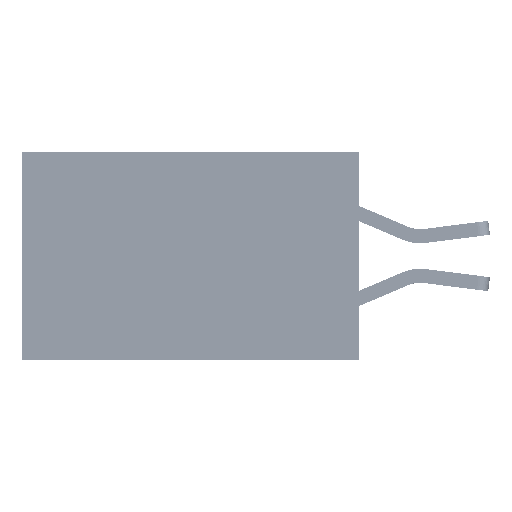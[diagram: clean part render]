
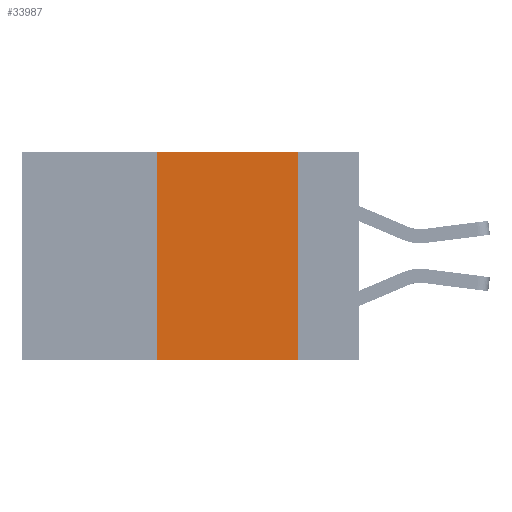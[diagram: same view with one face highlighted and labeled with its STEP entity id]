
A CAD part, left-side view. The second image highlights one B-rep face of the part: STEP entity #33987.
In plain terms, the highlighted planar face has unit normal (-1, 0, 0).
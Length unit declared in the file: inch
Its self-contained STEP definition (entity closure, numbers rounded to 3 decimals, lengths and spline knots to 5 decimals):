
#4740 = LINE ( 'NONE', #5862, #39469 ) ;
#4806 = LINE ( 'NONE', #19935, #34744 ) ;
#5862 = CARTESIAN_POINT ( 'NONE',  ( 0., 0.6, -0.37 ) ) ;
#6550 = CARTESIAN_POINT ( 'NONE',  ( 0., 0.11, -0.37 ) ) ;
#7282 = VECTOR ( 'NONE', #29513, 39.37008 ) ;
#7959 = VERTEX_POINT ( 'NONE', #6550 ) ;
#8239 = CARTESIAN_POINT ( 'NONE',  ( 0., 0.36, 0. ) ) ;
#9688 = VECTOR ( 'NONE', #29973, 39.37008 ) ;
#13762 = VERTEX_POINT ( 'NONE', #41750 ) ;
#14531 = CARTESIAN_POINT ( 'NONE',  ( 0., 0.11, 0. ) ) ;
#14538 = ORIENTED_EDGE ( 'NONE', *, *, #48262, .F. ) ;
#15694 = AXIS2_PLACEMENT_3D ( 'NONE', #31731, #24053, #27893 ) ;
#19935 = CARTESIAN_POINT ( 'NONE',  ( 0., 0.6, 0. ) ) ;
#20183 = PLANE ( 'NONE',  #15694 ) ;
#22942 = ORIENTED_EDGE ( 'NONE', *, *, #47443, .F. ) ;
#24053 = DIRECTION ( 'NONE',  ( 1., 0., 0. ) ) ;
#26331 = ORIENTED_EDGE ( 'NONE', *, *, #41389, .T. ) ;
#26552 = FACE_OUTER_BOUND ( 'NONE', #44270, .T. ) ;
#27893 = DIRECTION ( 'NONE',  ( 0., 0., -1. ) ) ;
#29513 = DIRECTION ( 'NONE',  ( 0., 0., 1. ) ) ;
#29973 = DIRECTION ( 'NONE',  ( 0., 0., -1. ) ) ;
#31731 = CARTESIAN_POINT ( 'NONE',  ( 0., 0.6, 0. ) ) ;
#32965 = VERTEX_POINT ( 'NONE', #38809 ) ;
#33987 = ADVANCED_FACE ( 'NONE', ( #26552 ), #20183, .F. ) ;
#34744 = VECTOR ( 'NONE', #38861, 39.37008 ) ;
#35955 = ORIENTED_EDGE ( 'NONE', *, *, #46121, .F. ) ;
#38809 = CARTESIAN_POINT ( 'NONE',  ( 0., 0.11, 0. ) ) ;
#38861 = DIRECTION ( 'NONE',  ( 0., -1., 0. ) ) ;
#39035 = LINE ( 'NONE', #48806, #7282 ) ;
#39469 = VECTOR ( 'NONE', #40149, 39.37008 ) ;
#40149 = DIRECTION ( 'NONE',  ( 0., -1., 0. ) ) ;
#41389 = EDGE_CURVE ( 'NONE', #13762, #7959, #4740, .T. ) ;
#41750 = CARTESIAN_POINT ( 'NONE',  ( 0., 0.36, -0.37 ) ) ;
#42003 = LINE ( 'NONE', #14531, #9688 ) ;
#43962 = VERTEX_POINT ( 'NONE', #8239 ) ;
#44270 = EDGE_LOOP ( 'NONE', ( #35955, #14538, #22942, #26331 ) ) ;
#46121 = EDGE_CURVE ( 'NONE', #32965, #7959, #42003, .T. ) ;
#47443 = EDGE_CURVE ( 'NONE', #13762, #43962, #39035, .T. ) ;
#48262 = EDGE_CURVE ( 'NONE', #43962, #32965, #4806, .T. ) ;
#48806 = CARTESIAN_POINT ( 'NONE',  ( 0., 0.36, 0. ) ) ;
